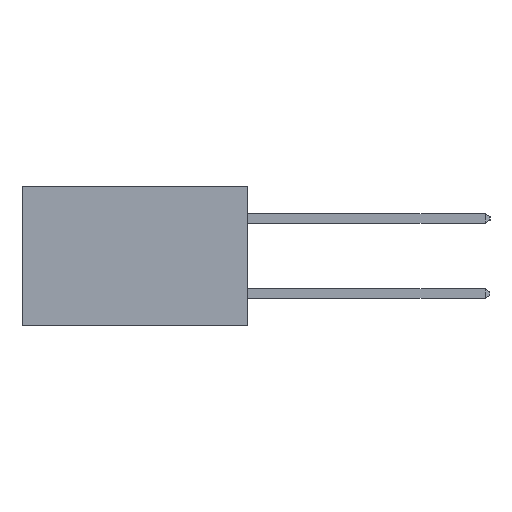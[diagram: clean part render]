
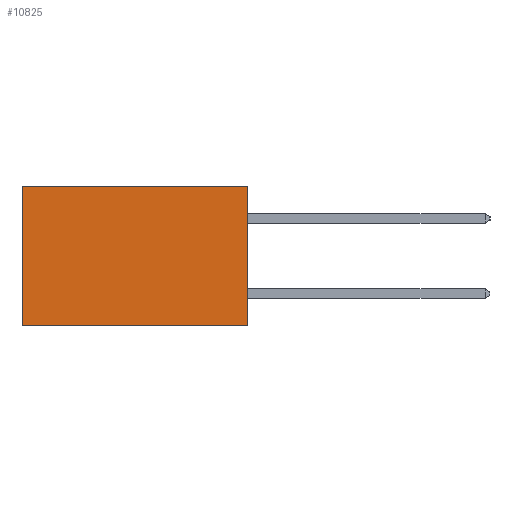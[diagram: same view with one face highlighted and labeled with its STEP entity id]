
A CAD part, left-side view. The second image highlights one B-rep face of the part: STEP entity #10825.
In plain terms, the highlighted planar face has unit normal (-1, 0, 0).
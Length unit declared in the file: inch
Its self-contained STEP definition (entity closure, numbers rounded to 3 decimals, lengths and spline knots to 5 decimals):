
#248 = VERTEX_POINT ( 'NONE', #6108 ) ;
#920 = VERTEX_POINT ( 'NONE', #10605 ) ;
#1123 = ORIENTED_EDGE ( 'NONE', *, *, #1989, .T. ) ;
#1257 = LINE ( 'NONE', #11472, #17233 ) ;
#1288 = VECTOR ( 'NONE', #1586, 39.37008 ) ;
#1586 = DIRECTION ( 'NONE',  ( 0., 1., 0. ) ) ;
#1989 = EDGE_CURVE ( 'NONE', #12319, #920, #8444, .T. ) ;
#3456 = CARTESIAN_POINT ( 'NONE',  ( 0.298, 0.6, 0. ) ) ;
#4999 = CARTESIAN_POINT ( 'NONE',  ( 0.298, 0., 0. ) ) ;
#5969 = FACE_OUTER_BOUND ( 'NONE', #11714, .T. ) ;
#6108 = CARTESIAN_POINT ( 'NONE',  ( 0.298, 0., -0.37 ) ) ;
#7640 = CARTESIAN_POINT ( 'NONE',  ( 0.298, 0., 0. ) ) ;
#8407 = DIRECTION ( 'NONE',  ( 0., 0., -1. ) ) ;
#8444 = LINE ( 'NONE', #10493, #15845 ) ;
#9160 = DIRECTION ( 'NONE',  ( 0., 0., -1. ) ) ;
#9397 = VERTEX_POINT ( 'NONE', #7640 ) ;
#9556 = DIRECTION ( 'NONE',  ( 0., 0., -1. ) ) ;
#10493 = CARTESIAN_POINT ( 'NONE',  ( 0.298, 0.6, 0. ) ) ;
#10605 = CARTESIAN_POINT ( 'NONE',  ( 0.298, 0.6, -0.37 ) ) ;
#10654 = ORIENTED_EDGE ( 'NONE', *, *, #14051, .T. ) ;
#10825 = ADVANCED_FACE ( 'NONE', ( #5969 ), #16924, .F. ) ;
#11472 = CARTESIAN_POINT ( 'NONE',  ( 0.298, 0., 0. ) ) ;
#11714 = EDGE_LOOP ( 'NONE', ( #1123, #17758, #13485, #10654 ) ) ;
#12319 = VERTEX_POINT ( 'NONE', #3456 ) ;
#13403 = LINE ( 'NONE', #16574, #1288 ) ;
#13485 = ORIENTED_EDGE ( 'NONE', *, *, #18910, .F. ) ;
#13532 = EDGE_CURVE ( 'NONE', #248, #920, #13403, .T. ) ;
#14051 = EDGE_CURVE ( 'NONE', #9397, #12319, #18835, .T. ) ;
#14197 = CARTESIAN_POINT ( 'NONE',  ( 0.298, 0., 0. ) ) ;
#15646 = DIRECTION ( 'NONE',  ( 0., 1., 0. ) ) ;
#15845 = VECTOR ( 'NONE', #9160, 39.37008 ) ;
#16574 = CARTESIAN_POINT ( 'NONE',  ( 0.298, 0., -0.37 ) ) ;
#16924 = PLANE ( 'NONE',  #17898 ) ;
#17233 = VECTOR ( 'NONE', #8407, 39.37008 ) ;
#17758 = ORIENTED_EDGE ( 'NONE', *, *, #13532, .F. ) ;
#17898 = AXIS2_PLACEMENT_3D ( 'NONE', #4999, #18373, #9556 ) ;
#18365 = VECTOR ( 'NONE', #15646, 39.37008 ) ;
#18373 = DIRECTION ( 'NONE',  ( 1., 0., 0. ) ) ;
#18835 = LINE ( 'NONE', #14197, #18365 ) ;
#18910 = EDGE_CURVE ( 'NONE', #9397, #248, #1257, .T. ) ;
